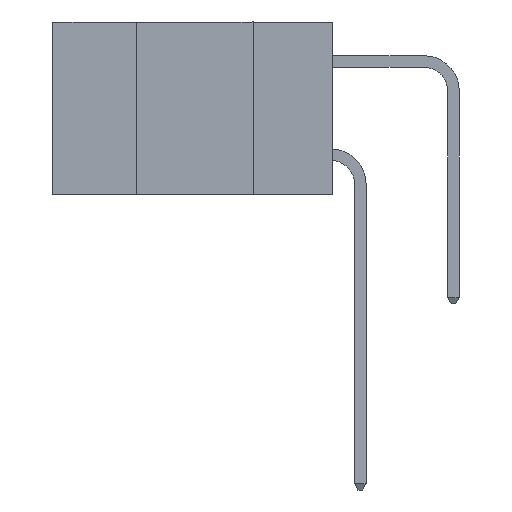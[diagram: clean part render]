
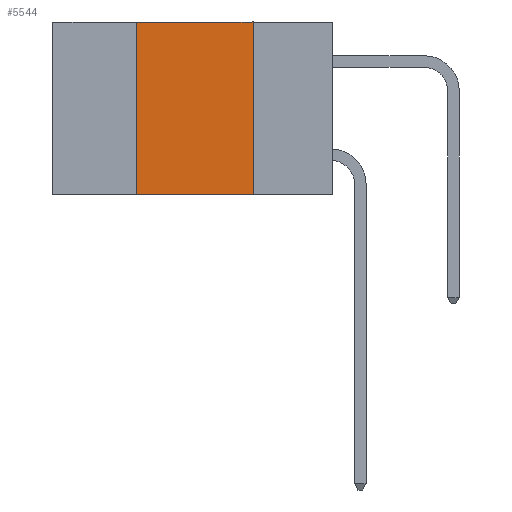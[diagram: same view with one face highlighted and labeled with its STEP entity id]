
A CAD part, left-side view. The second image highlights one B-rep face of the part: STEP entity #5544.
In plain terms, the highlighted planar face has unit normal (-1, 0, 0).
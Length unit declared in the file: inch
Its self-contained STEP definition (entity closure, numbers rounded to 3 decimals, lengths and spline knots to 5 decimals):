
#760 = CARTESIAN_POINT ( 'NONE',  ( 0., 0.42, 0. ) ) ;
#975 = EDGE_CURVE ( 'NONE', #3601, #4503, #1324, .T. ) ;
#1028 = DIRECTION ( 'NONE',  ( 0., 0., -1. ) ) ;
#1165 = CARTESIAN_POINT ( 'NONE',  ( 0., 0.17, -0.37 ) ) ;
#1324 = LINE ( 'NONE', #1165, #12575 ) ;
#1391 = CARTESIAN_POINT ( 'NONE',  ( 0., 0.42, -0.37 ) ) ;
#1956 = EDGE_CURVE ( 'NONE', #12778, #8538, #3175, .T. ) ;
#2137 = VECTOR ( 'NONE', #6493, 39.37008 ) ;
#2751 = CARTESIAN_POINT ( 'NONE',  ( 0., 0.17, -0.37 ) ) ;
#2990 = FACE_OUTER_BOUND ( 'NONE', #8152, .T. ) ;
#3175 = LINE ( 'NONE', #1391, #5706 ) ;
#3341 = CARTESIAN_POINT ( 'NONE',  ( 0., 0.17, 0. ) ) ;
#3601 = VERTEX_POINT ( 'NONE', #3341 ) ;
#4503 = VERTEX_POINT ( 'NONE', #2751 ) ;
#5419 = CARTESIAN_POINT ( 'NONE',  ( 0., 0.6, 0. ) ) ;
#5523 = ORIENTED_EDGE ( 'NONE', *, *, #975, .F. ) ;
#5544 = ADVANCED_FACE ( 'NONE', ( #2990 ), #11669, .F. ) ;
#5610 = DIRECTION ( 'NONE',  ( 0., 0., 1. ) ) ;
#5706 = VECTOR ( 'NONE', #5610, 39.37008 ) ;
#5755 = DIRECTION ( 'NONE',  ( 0., -1., 0. ) ) ;
#5863 = ORIENTED_EDGE ( 'NONE', *, *, #10528, .F. ) ;
#6304 = CARTESIAN_POINT ( 'NONE',  ( 0., 0.42, -0.37 ) ) ;
#6458 = AXIS2_PLACEMENT_3D ( 'NONE', #5419, #12707, #6501 ) ;
#6493 = DIRECTION ( 'NONE',  ( 0., -1., 0. ) ) ;
#6501 = DIRECTION ( 'NONE',  ( 0., 0., -1. ) ) ;
#7107 = EDGE_CURVE ( 'NONE', #12778, #4503, #9443, .T. ) ;
#8152 = EDGE_LOOP ( 'NONE', ( #5523, #5863, #10929, #13185 ) ) ;
#8213 = LINE ( 'NONE', #10641, #2137 ) ;
#8538 = VERTEX_POINT ( 'NONE', #760 ) ;
#9443 = LINE ( 'NONE', #13022, #11521 ) ;
#10528 = EDGE_CURVE ( 'NONE', #8538, #3601, #8213, .T. ) ;
#10641 = CARTESIAN_POINT ( 'NONE',  ( 0., 0.6, 0. ) ) ;
#10929 = ORIENTED_EDGE ( 'NONE', *, *, #1956, .F. ) ;
#11521 = VECTOR ( 'NONE', #5755, 39.37008 ) ;
#11669 = PLANE ( 'NONE',  #6458 ) ;
#12575 = VECTOR ( 'NONE', #1028, 39.37008 ) ;
#12707 = DIRECTION ( 'NONE',  ( 1., 0., 0. ) ) ;
#12778 = VERTEX_POINT ( 'NONE', #6304 ) ;
#13022 = CARTESIAN_POINT ( 'NONE',  ( 0., 0.6, -0.37 ) ) ;
#13185 = ORIENTED_EDGE ( 'NONE', *, *, #7107, .T. ) ;
